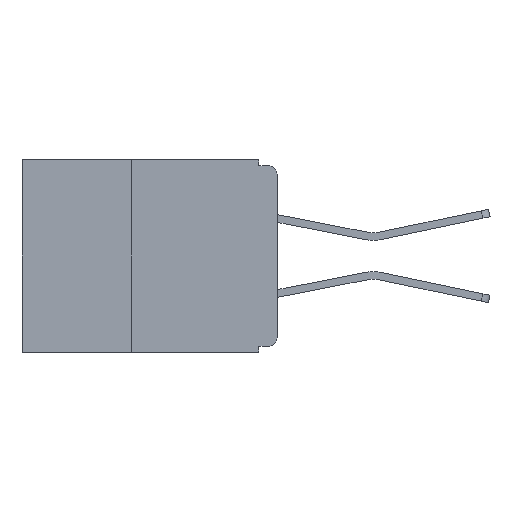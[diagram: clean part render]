
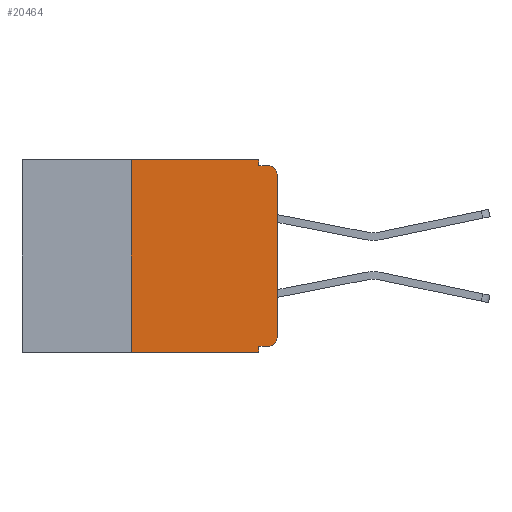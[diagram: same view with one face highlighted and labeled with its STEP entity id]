
A CAD part, left-side view. The second image highlights one B-rep face of the part: STEP entity #20464.
In plain terms, the highlighted planar face has unit normal (-1, 0, 0).
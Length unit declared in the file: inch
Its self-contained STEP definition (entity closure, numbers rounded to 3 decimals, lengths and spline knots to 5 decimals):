
#378 = DIRECTION ( 'NONE',  ( -1., 0., 0. ) ) ;
#1200 = DIRECTION ( 'NONE',  ( 0., -1., 0. ) ) ;
#1291 = CARTESIAN_POINT ( 'NONE',  ( 0., 0., -0.025 ) ) ;
#1355 = LINE ( 'NONE', #14822, #5608 ) ;
#1419 = VECTOR ( 'NONE', #16131, 39.37008 ) ;
#1433 = CARTESIAN_POINT ( 'NONE',  ( 0., 0., -0.305 ) ) ;
#1619 = PLANE ( 'NONE',  #4739 ) ;
#1642 = EDGE_CURVE ( 'NONE', #9787, #2197, #6961, .T. ) ;
#1886 = ORIENTED_EDGE ( 'NONE', *, *, #2367, .T. ) ;
#1929 = LINE ( 'NONE', #15256, #1419 ) ;
#2197 = VERTEX_POINT ( 'NONE', #19551 ) ;
#2198 = CARTESIAN_POINT ( 'NONE',  ( 0., 0.031, 0. ) ) ;
#2225 = EDGE_CURVE ( 'NONE', #7294, #12731, #8676, .T. ) ;
#2359 = LINE ( 'NONE', #4586, #18467 ) ;
#2367 = EDGE_CURVE ( 'NONE', #7294, #11234, #1929, .T. ) ;
#3040 = AXIS2_PLACEMENT_3D ( 'NONE', #10036, #378, #11666 ) ;
#3090 = LINE ( 'NONE', #10842, #11653 ) ;
#3251 = DIRECTION ( 'NONE',  ( 1., 0., 0. ) ) ;
#3534 = VERTEX_POINT ( 'NONE', #5717 ) ;
#4061 = AXIS2_PLACEMENT_3D ( 'NONE', #13015, #12595, #20560 ) ;
#4119 = VERTEX_POINT ( 'NONE', #13216 ) ;
#4301 = CARTESIAN_POINT ( 'NONE',  ( 0., 0.015, -0.32 ) ) ;
#4463 = VECTOR ( 'NONE', #16111, 39.37008 ) ;
#4586 = CARTESIAN_POINT ( 'NONE',  ( 0., 0.031, -0.33 ) ) ;
#4739 = AXIS2_PLACEMENT_3D ( 'NONE', #11259, #3251, #14511 ) ;
#5171 = DIRECTION ( 'NONE',  ( 0., 0., -1. ) ) ;
#5608 = VECTOR ( 'NONE', #5171, 39.37008 ) ;
#5717 = CARTESIAN_POINT ( 'NONE',  ( 0., 0.031, -0.32 ) ) ;
#6170 = DIRECTION ( 'NONE',  ( 0., 0., -1. ) ) ;
#6781 = EDGE_CURVE ( 'NONE', #19787, #9787, #17183, .T. ) ;
#6961 = CIRCLE ( 'NONE', #4061, 0.015 ) ;
#7277 = EDGE_CURVE ( 'NONE', #4119, #2197, #7570, .T. ) ;
#7294 = VERTEX_POINT ( 'NONE', #8009 ) ;
#7401 = CIRCLE ( 'NONE', #3040, 0.015 ) ;
#7570 = LINE ( 'NONE', #8267, #15660 ) ;
#7729 = VERTEX_POINT ( 'NONE', #4301 ) ;
#7941 = VECTOR ( 'NONE', #11746, 39.37008 ) ;
#8009 = CARTESIAN_POINT ( 'NONE',  ( 0., 0.25, -0.33 ) ) ;
#8126 = ORIENTED_EDGE ( 'NONE', *, *, #6781, .T. ) ;
#8220 = DIRECTION ( 'NONE',  ( 0., -1., 0. ) ) ;
#8267 = CARTESIAN_POINT ( 'NONE',  ( 0., 0., -0.01 ) ) ;
#8397 = ORIENTED_EDGE ( 'NONE', *, *, #7277, .F. ) ;
#8635 = ORIENTED_EDGE ( 'NONE', *, *, #12252, .F. ) ;
#8676 = LINE ( 'NONE', #15946, #4463 ) ;
#9787 = VERTEX_POINT ( 'NONE', #1291 ) ;
#10036 = CARTESIAN_POINT ( 'NONE',  ( 0., 0.015, -0.305 ) ) ;
#10105 = CARTESIAN_POINT ( 'NONE',  ( 0., 0.031, -0.33 ) ) ;
#10130 = CARTESIAN_POINT ( 'NONE',  ( 0., 0., -0.32 ) ) ;
#10614 = EDGE_CURVE ( 'NONE', #7729, #3534, #20757, .T. ) ;
#10842 = CARTESIAN_POINT ( 'NONE',  ( 0., 0.437, 0. ) ) ;
#11234 = VERTEX_POINT ( 'NONE', #10105 ) ;
#11259 = CARTESIAN_POINT ( 'NONE',  ( 0., 0.437, 0. ) ) ;
#11653 = VECTOR ( 'NONE', #1200, 39.37008 ) ;
#11666 = DIRECTION ( 'NONE',  ( 0., 0., -1. ) ) ;
#11746 = DIRECTION ( 'NONE',  ( 0., 1., 0. ) ) ;
#12237 = ORIENTED_EDGE ( 'NONE', *, *, #15320, .F. ) ;
#12252 = EDGE_CURVE ( 'NONE', #3534, #11234, #2359, .T. ) ;
#12581 = EDGE_LOOP ( 'NONE', ( #8126, #18236, #8397, #13224, #12237, #17492, #1886, #8635, #12982, #16011 ) ) ;
#12595 = DIRECTION ( 'NONE',  ( -1., 0., 0. ) ) ;
#12731 = VERTEX_POINT ( 'NONE', #20032 ) ;
#12982 = ORIENTED_EDGE ( 'NONE', *, *, #10614, .F. ) ;
#13015 = CARTESIAN_POINT ( 'NONE',  ( 0., 0.015, -0.025 ) ) ;
#13216 = CARTESIAN_POINT ( 'NONE',  ( 0., 0.031, -0.01 ) ) ;
#13224 = ORIENTED_EDGE ( 'NONE', *, *, #14358, .F. ) ;
#13702 = CARTESIAN_POINT ( 'NONE',  ( 0., 0., 0. ) ) ;
#13743 = DIRECTION ( 'NONE',  ( 0., 0., 1. ) ) ;
#13822 = EDGE_CURVE ( 'NONE', #7729, #19787, #7401, .T. ) ;
#14358 = EDGE_CURVE ( 'NONE', #16792, #4119, #1355, .T. ) ;
#14511 = DIRECTION ( 'NONE',  ( 0., 0., -1. ) ) ;
#14822 = CARTESIAN_POINT ( 'NONE',  ( 0., 0.031, 0. ) ) ;
#15256 = CARTESIAN_POINT ( 'NONE',  ( 0., 0.437, -0.33 ) ) ;
#15320 = EDGE_CURVE ( 'NONE', #12731, #16792, #3090, .T. ) ;
#15389 = FACE_OUTER_BOUND ( 'NONE', #12581, .T. ) ;
#15660 = VECTOR ( 'NONE', #8220, 39.37008 ) ;
#15946 = CARTESIAN_POINT ( 'NONE',  ( 0., 0.25, -0.33 ) ) ;
#16011 = ORIENTED_EDGE ( 'NONE', *, *, #13822, .T. ) ;
#16111 = DIRECTION ( 'NONE',  ( 0., 0., 1. ) ) ;
#16131 = DIRECTION ( 'NONE',  ( 0., -1., 0. ) ) ;
#16687 = VECTOR ( 'NONE', #13743, 39.37008 ) ;
#16792 = VERTEX_POINT ( 'NONE', #2198 ) ;
#17183 = LINE ( 'NONE', #13702, #16687 ) ;
#17492 = ORIENTED_EDGE ( 'NONE', *, *, #2225, .F. ) ;
#18236 = ORIENTED_EDGE ( 'NONE', *, *, #1642, .T. ) ;
#18467 = VECTOR ( 'NONE', #6170, 39.37008 ) ;
#19551 = CARTESIAN_POINT ( 'NONE',  ( 0., 0.015, -0.01 ) ) ;
#19787 = VERTEX_POINT ( 'NONE', #1433 ) ;
#20032 = CARTESIAN_POINT ( 'NONE',  ( 0., 0.25, 0. ) ) ;
#20464 = ADVANCED_FACE ( 'NONE', ( #15389 ), #1619, .F. ) ;
#20560 = DIRECTION ( 'NONE',  ( 0., 0., -1. ) ) ;
#20757 = LINE ( 'NONE', #10130, #7941 ) ;
